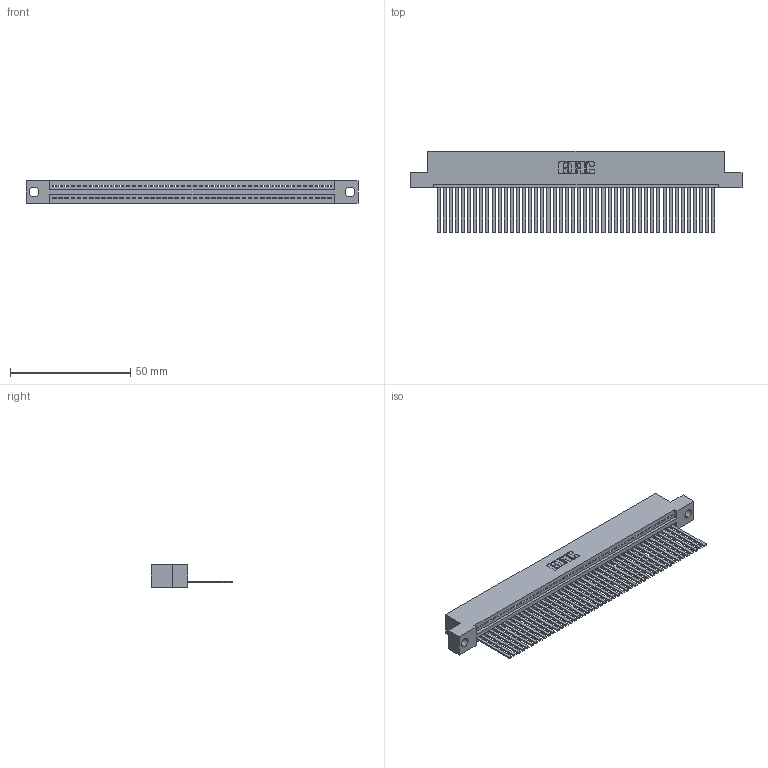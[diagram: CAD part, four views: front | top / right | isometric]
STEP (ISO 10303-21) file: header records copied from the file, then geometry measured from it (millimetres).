
FILE_DESCRIPTION (( 'STEP AP203' ), '1' );
FILE_NAME ('345-046-544-104.STEP', '2019-10-09T00:25:44', ( '' ), ( '' ), 'SwSTEP 2.0', 'SolidWorks 2016', '' );
FILE_SCHEMA (( 'CONFIG_CONTROL_DESIGN' ));
Length unit declared in the file: inch
Products named in the file (3): 345-292-001_345-293-144; 345-046-544-104; 345 Part_Flush Mounting Lugs - 0.156 Dia-TH
Assembly tree (47 placements, depth 2):
  345-046-544-104
    345 Part_Flush Mounting Lugs - 0.156 Dia-TH
    345-292-001_345-293-144  x46
Bounding box: 138.05 x 33.96 x 9.4 mm (x, y, z)
Volume: 13589.7 mm3; surface area: 19521.9 mm2
Topology: 47 solids, 47 shells, 2518 faces, 7609 edges, 5010 vertices
Faces by surface type: plane 1736, cylinder 782
Entity records: 33901 total; most frequent: CARTESIAN_POINT 5878, ORIENTED_EDGE 5858, DIRECTION 5125, EDGE_CURVE 2929, VECTOR 2617, LINE 2617, VERTEX_POINT 1950, AXIS2_PLACEMENT_3D 1254
